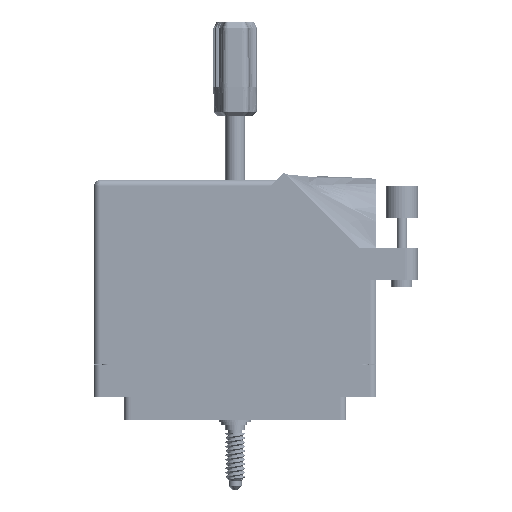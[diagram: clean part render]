
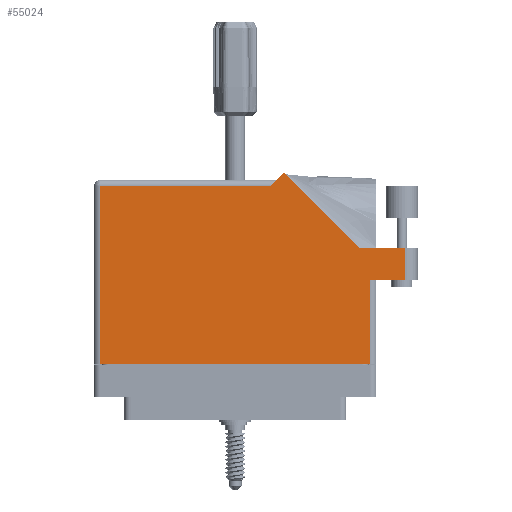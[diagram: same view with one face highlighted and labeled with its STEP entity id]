
A CAD part, front view. The second image highlights one B-rep face of the part: STEP entity #55024.
In plain terms, the highlighted face is planar.
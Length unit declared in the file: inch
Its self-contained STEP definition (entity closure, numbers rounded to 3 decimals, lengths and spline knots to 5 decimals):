
#2172 = VECTOR ( 'NONE', #13834, 39.37008 ) ;
#3299 = ORIENTED_EDGE ( 'NONE', *, *, #44489, .T. ) ;
#3955 = LINE ( 'NONE', #63698, #58242 ) ;
#4539 = CARTESIAN_POINT ( 'NONE',  ( -1.297, -0.1, 0.617 ) ) ;
#6639 = VECTOR ( 'NONE', #31330, 39.37008 ) ;
#8142 = ORIENTED_EDGE ( 'NONE', *, *, #85154, .T. ) ;
#9200 = DIRECTION ( 'NONE',  ( 0., 1., 0. ) ) ;
#11111 = CARTESIAN_POINT ( 'NONE',  ( 1.759, 1.022, 0.617 ) ) ;
#12106 = DIRECTION ( 'NONE',  ( -1., 0., 0. ) ) ;
#12749 = EDGE_CURVE ( 'NONE', #37108, #27713, #45067, .T. ) ;
#13515 = EDGE_CURVE ( 'NONE', #73480, #37108, #74820, .T. ) ;
#13834 = DIRECTION ( 'NONE',  ( -0.707, 0.707, 0. ) ) ;
#14642 = EDGE_CURVE ( 'NONE', #45558, #37237, #62099, .T. ) ;
#23847 = CARTESIAN_POINT ( 'NONE',  ( 0.337, 1.613, 0.617 ) ) ;
#24659 = EDGE_CURVE ( 'NONE', #80996, #43206, #75581, .T. ) ;
#25135 = ORIENTED_EDGE ( 'NONE', *, *, #12749, .T. ) ;
#25168 = VECTOR ( 'NONE', #82761, 39.37008 ) ;
#25468 = EDGE_CURVE ( 'NONE', #27713, #34443, #64710, .T. ) ;
#25704 = CARTESIAN_POINT ( 'NONE',  ( 1.19342, 1.022, 0.617 ) ) ;
#26125 = CARTESIAN_POINT ( 'NONE',  ( 1.297, 0.715, 0.617 ) ) ;
#27713 = VERTEX_POINT ( 'NONE', #56422 ) ;
#28285 = EDGE_CURVE ( 'NONE', #37237, #32998, #66448, .T. ) ;
#30202 = ORIENTED_EDGE ( 'NONE', *, *, #13515, .T. ) ;
#30307 = DIRECTION ( 'NONE',  ( 1., 0., 0. ) ) ;
#31214 = VECTOR ( 'NONE', #83044, 39.37008 ) ;
#31330 = DIRECTION ( 'NONE',  ( 0., -1., 0. ) ) ;
#32998 = VERTEX_POINT ( 'NONE', #49673 ) ;
#34443 = VERTEX_POINT ( 'NONE', #66235 ) ;
#34980 = CARTESIAN_POINT ( 'NONE',  ( 1.634, 0.715, 0.617 ) ) ;
#37108 = VERTEX_POINT ( 'NONE', #23847 ) ;
#37237 = VERTEX_POINT ( 'NONE', #59412 ) ;
#37924 = DIRECTION ( 'NONE',  ( -1., 0., 0. ) ) ;
#40035 = CARTESIAN_POINT ( 'NONE',  ( -1.359, 1.675, 0.617 ) ) ;
#40995 = DIRECTION ( 'NONE',  ( -0.707, -0.707, 0. ) ) ;
#42134 = ORIENTED_EDGE ( 'NONE', *, *, #14642, .T. ) ;
#43206 = VERTEX_POINT ( 'NONE', #26125 ) ;
#44489 = EDGE_CURVE ( 'NONE', #32998, #73480, #81072, .T. ) ;
#45067 = LINE ( 'NONE', #71886, #79843 ) ;
#45324 = DIRECTION ( 'NONE',  ( 0., 0., -1. ) ) ;
#45558 = VERTEX_POINT ( 'NONE', #34980 ) ;
#48014 = CARTESIAN_POINT ( 'NONE',  ( 0.399, 1.675, 0.617 ) ) ;
#49245 = VECTOR ( 'NONE', #40995, 39.37008 ) ;
#49673 = CARTESIAN_POINT ( 'NONE',  ( 1.19342, 1.022, 0.617 ) ) ;
#55024 = ADVANCED_FACE ( 'NONE', ( #65517 ), #60235, .F. ) ;
#56204 = CARTESIAN_POINT ( 'NONE',  ( 1.359, 0.715, 0.617 ) ) ;
#56422 = CARTESIAN_POINT ( 'NONE',  ( -1.297, 1.613, 0.617 ) ) ;
#58242 = VECTOR ( 'NONE', #30307, 39.37008 ) ;
#59412 = CARTESIAN_POINT ( 'NONE',  ( 1.634, 1.022, 0.617 ) ) ;
#60235 = PLANE ( 'NONE',  #81854 ) ;
#62099 = LINE ( 'NONE', #63392, #25168 ) ;
#62794 = LINE ( 'NONE', #56204, #31214 ) ;
#63392 = CARTESIAN_POINT ( 'NONE',  ( 1.634, 1.022, 0.617 ) ) ;
#63698 = CARTESIAN_POINT ( 'NONE',  ( -1.359, -0.1, 0.617 ) ) ;
#64710 = LINE ( 'NONE', #4539, #6639 ) ;
#65517 = FACE_OUTER_BOUND ( 'NONE', #68997, .T. ) ;
#66235 = CARTESIAN_POINT ( 'NONE',  ( -1.297, -0.1, 0.617 ) ) ;
#66448 = LINE ( 'NONE', #11111, #81354 ) ;
#68997 = EDGE_LOOP ( 'NONE', ( #8142, #42134, #85684, #3299, #30202, #25135, #81089, #79002, #85123 ) ) ;
#70467 = EDGE_CURVE ( 'NONE', #34443, #80996, #3955, .T. ) ;
#71886 = CARTESIAN_POINT ( 'NONE',  ( -1.359, 1.613, 0.617 ) ) ;
#72133 = DIRECTION ( 'NONE',  ( -1., 0., 0. ) ) ;
#72325 = CARTESIAN_POINT ( 'NONE',  ( 1.297, -0.1, 0.617 ) ) ;
#73480 = VERTEX_POINT ( 'NONE', #82601 ) ;
#74820 = LINE ( 'NONE', #48014, #49245 ) ;
#75581 = LINE ( 'NONE', #76444, #83937 ) ;
#76444 = CARTESIAN_POINT ( 'NONE',  ( 1.297, 0.715, 0.617 ) ) ;
#79002 = ORIENTED_EDGE ( 'NONE', *, *, #70467, .T. ) ;
#79843 = VECTOR ( 'NONE', #12106, 39.37008 ) ;
#80996 = VERTEX_POINT ( 'NONE', #72325 ) ;
#81072 = LINE ( 'NONE', #25704, #2172 ) ;
#81089 = ORIENTED_EDGE ( 'NONE', *, *, #25468, .T. ) ;
#81354 = VECTOR ( 'NONE', #37924, 39.37008 ) ;
#81854 = AXIS2_PLACEMENT_3D ( 'NONE', #40035, #45324, #72133 ) ;
#82601 = CARTESIAN_POINT ( 'NONE',  ( 0.46971, 1.74571, 0.617 ) ) ;
#82761 = DIRECTION ( 'NONE',  ( 0., 1., 0. ) ) ;
#83044 = DIRECTION ( 'NONE',  ( 1., 0., 0. ) ) ;
#83937 = VECTOR ( 'NONE', #9200, 39.37008 ) ;
#85123 = ORIENTED_EDGE ( 'NONE', *, *, #24659, .T. ) ;
#85154 = EDGE_CURVE ( 'NONE', #43206, #45558, #62794, .T. ) ;
#85684 = ORIENTED_EDGE ( 'NONE', *, *, #28285, .T. ) ;
